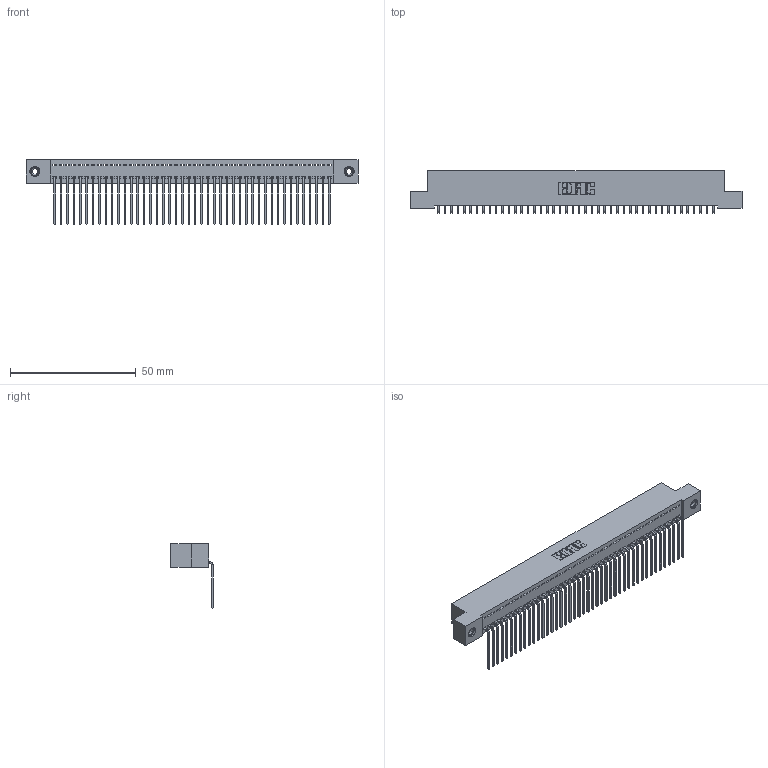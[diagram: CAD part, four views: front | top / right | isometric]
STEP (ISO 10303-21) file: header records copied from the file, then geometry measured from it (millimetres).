
FILE_DESCRIPTION (( 'STEP AP203' ), '1' );
FILE_NAME ('392-044-559-108.STEP', '2019-10-07T22:45:33', ( '' ), ( '' ), 'SwSTEP 2.0', 'SolidWorks 2016', '' );
FILE_SCHEMA (( 'CONFIG_CONTROL_DESIGN' ));
Length unit declared in the file: inch
Products named in the file (4): 345-250-001_345-250-003-102; 392-044-559-108; 342 Part_TI; 345-292-001_558 559 Tail - 1
Assembly tree (47 placements, depth 2):
  392-044-559-108
    342 Part_TI
    345-292-001_558 559 Tail - 1  x44
    345-250-001_345-250-003-102  x2
Bounding box: 132.08 x 16.83 x 25.78 mm (x, y, z)
Volume: 11729.1 mm3; surface area: 18111.3 mm2
Topology: 47 solids, 47 shells, 2810 faces, 8443 edges, 5562 vertices
Faces by surface type: plane 2034, cylinder 760, cone 12, torus 4
Entity records: 27778 total; most frequent: CARTESIAN_POINT 4773, ORIENTED_EDGE 4746, DIRECTION 4055, EDGE_CURVE 2373, LINE 2225, VECTOR 2225, VERTEX_POINT 1576, AXIS2_PLACEMENT_3D 915
